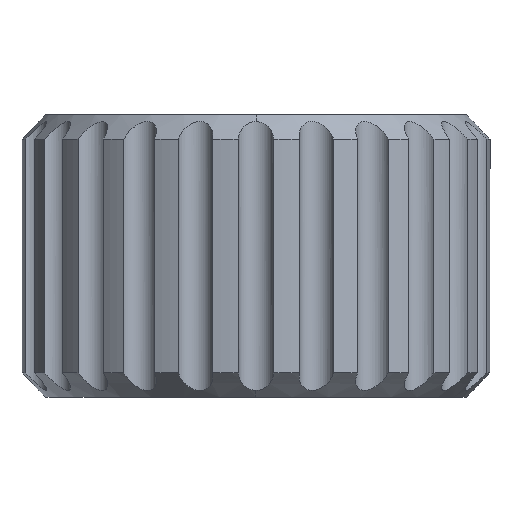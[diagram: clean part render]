
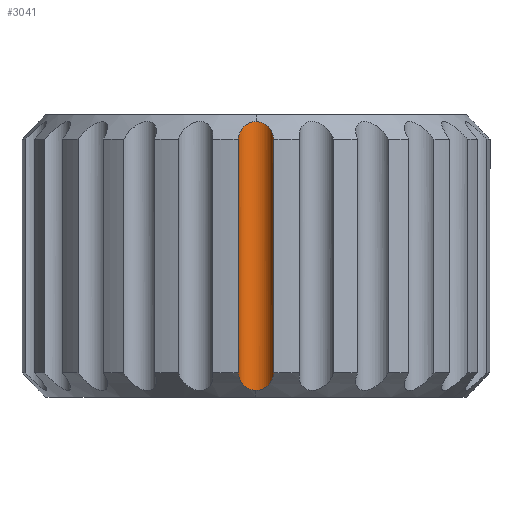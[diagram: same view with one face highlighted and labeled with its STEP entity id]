
A CAD part, front view. The second image highlights one B-rep face of the part: STEP entity #3041.
In plain terms, the highlighted cylindrical face has radius 0.635 mm (diameter 1.27 mm), a partial arc.
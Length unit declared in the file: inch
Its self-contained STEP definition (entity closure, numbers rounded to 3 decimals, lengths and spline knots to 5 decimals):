
#91 = CARTESIAN_POINT ( 'NONE',  ( -0.02498, -0.33124, -0.18272 ) ) ;
#121 = CARTESIAN_POINT ( 'NONE',  ( -0.02498, -0.33124, 0.14791 ) ) ;
#126 = CARTESIAN_POINT ( 'NONE',  ( 0., -0.30719, -0.20772 ) ) ;
#438 = CARTESIAN_POINT ( 'NONE',  ( -0.02281, -0.32026, -0.19387 ) ) ;
#469 = CARTESIAN_POINT ( 'NONE',  ( 0.00777, -0.30816, -0.20667 ) ) ;
#519 = DIRECTION ( 'NONE',  ( 0., 0., 1. ) ) ;
#771 = CARTESIAN_POINT ( 'NONE',  ( -0.0039, -0.30719, -0.20772 ) ) ;
#817 = CARTESIAN_POINT ( 'NONE',  ( -0.01414, -0.31127, -0.20334 ) ) ;
#821 = LINE ( 'NONE', #4590, #1552 ) ;
#883 = CARTESIAN_POINT ( 'NONE',  ( 0.02498, -0.33124, -0.18272 ) ) ;
#994 = CARTESIAN_POINT ( 'NONE',  ( -0.02498, -0.33124, 0.14791 ) ) ;
#1074 = ORIENTED_EDGE ( 'NONE', *, *, #4214, .T. ) ;
#1167 = CARTESIAN_POINT ( 'NONE',  ( -0.01673, -0.31336, -0.20111 ) ) ;
#1181 = CARTESIAN_POINT ( 'NONE',  ( 0.0039, -0.30719, 0.17291 ) ) ;
#1206 = VERTEX_POINT ( 'NONE', #91 ) ;
#1215 = CARTESIAN_POINT ( 'NONE',  ( 0., -0.30719, 0.17291 ) ) ;
#1312 = CARTESIAN_POINT ( 'NONE',  ( -0.02229, -0.32053, 0.15879 ) ) ;
#1376 = B_SPLINE_CURVE_WITH_KNOTS ( 'NONE', 3,
 ( #121, #2513, #2101, #1312, #4493, #3265, #2468, #2889, #3682, #3309 ),
 .UNSPECIFIED., .F., .F.,
 ( 4, 2, 2, 2, 4 ),
 ( 0., 0.0003, 0.00059, 0.00089, 0.00118 ),
 .UNSPECIFIED. ) ;
#1388 = ORIENTED_EDGE ( 'NONE', *, *, #3994, .T. ) ;
#1552 = VECTOR ( 'NONE', #3367, 39.37008 ) ;
#1601 = CARTESIAN_POINT ( 'NONE',  ( 0.0078, -0.30817, 0.17184 ) ) ;
#1610 = CARTESIAN_POINT ( 'NONE',  ( 0., -0.30719, 0.17291 ) ) ;
#1615 = CARTESIAN_POINT ( 'NONE',  ( 0.01414, -0.31127, 0.16852 ) ) ;
#1696 = AXIS2_PLACEMENT_3D ( 'NONE', #3336, #4533, #2103 ) ;
#1806 = CARTESIAN_POINT ( 'NONE',  ( 0.02498, -0.33124, -0.18272 ) ) ;
#1908 = VECTOR ( 'NONE', #519, 39.37008 ) ;
#1911 = EDGE_CURVE ( 'NONE', #2261, #3254, #1376, .T. ) ;
#1951 = CARTESIAN_POINT ( 'NONE',  ( -0.02498, -0.33124, -0.18272 ) ) ;
#1966 = CARTESIAN_POINT ( 'NONE',  ( 0., -0.30719, -0.20772 ) ) ;
#1970 = CYLINDRICAL_SURFACE ( 'NONE', #1696, 0.025 ) ;
#1986 = VERTEX_POINT ( 'NONE', #1806 ) ;
#2101 = CARTESIAN_POINT ( 'NONE',  ( -0.02432, -0.32577, 0.15342 ) ) ;
#2103 = DIRECTION ( 'NONE',  ( 1., 0., 0. ) ) ;
#2135 = CARTESIAN_POINT ( 'NONE',  ( 0.02498, -0.33124, 0.14791 ) ) ;
#2177 = ORIENTED_EDGE ( 'NONE', *, *, #4088, .F. ) ;
#2261 = VERTEX_POINT ( 'NONE', #994 ) ;
#2353 = CARTESIAN_POINT ( 'NONE',  ( -0.02477, -0.32569, -0.18828 ) ) ;
#2402 = CARTESIAN_POINT ( 'NONE',  ( 0.02432, -0.32577, -0.18824 ) ) ;
#2422 = CARTESIAN_POINT ( 'NONE',  ( 0.02281, -0.32026, 0.15905 ) ) ;
#2468 = CARTESIAN_POINT ( 'NONE',  ( -0.01417, -0.31128, 0.1685 ) ) ;
#2469 = LINE ( 'NONE', #3967, #1908 ) ;
#2513 = CARTESIAN_POINT ( 'NONE',  ( -0.02488, -0.32846, 0.15069 ) ) ;
#2651 = VERTEX_POINT ( 'NONE', #126 ) ;
#2764 = EDGE_CURVE ( 'NONE', #3254, #4951, #3009, .T. ) ;
#2796 = CARTESIAN_POINT ( 'NONE',  ( 0.01673, -0.31336, 0.16629 ) ) ;
#2889 = CARTESIAN_POINT ( 'NONE',  ( -0.00777, -0.30816, 0.17185 ) ) ;
#3009 = B_SPLINE_CURVE_WITH_KNOTS ( 'NONE', 3,
 ( #1215, #1181, #1601, #1615, #2796, #2422, #4771, #4823 ),
 .UNSPECIFIED., .F., .F.,
 ( 4, 2, 2, 4 ),
 ( 0.00118, 0.00148, 0.00177, 0.00236 ),
 .UNSPECIFIED. ) ;
#3041 = ADVANCED_FACE ( 'NONE', ( #4818 ), #1970, .F. ) ;
#3176 = EDGE_CURVE ( 'NONE', #1986, #2651, #4265, .T. ) ;
#3191 = CARTESIAN_POINT ( 'NONE',  ( 0.0039, -0.30719, -0.20772 ) ) ;
#3213 = CARTESIAN_POINT ( 'NONE',  ( 0.02488, -0.32846, -0.1855 ) ) ;
#3254 = VERTEX_POINT ( 'NONE', #1610 ) ;
#3265 = CARTESIAN_POINT ( 'NONE',  ( -0.01675, -0.31338, 0.16627 ) ) ;
#3309 = CARTESIAN_POINT ( 'NONE',  ( 0., -0.30719, 0.17291 ) ) ;
#3336 = CARTESIAN_POINT ( 'NONE',  ( 0., -0.33219, -0.23962 ) ) ;
#3367 = DIRECTION ( 'NONE',  ( 0., 0., -1. ) ) ;
#3597 = CARTESIAN_POINT ( 'NONE',  ( 0.02229, -0.32053, -0.19361 ) ) ;
#3614 = CARTESIAN_POINT ( 'NONE',  ( 0., -0.30719, -0.20772 ) ) ;
#3646 = CARTESIAN_POINT ( 'NONE',  ( 0.02079, -0.31797, -0.19626 ) ) ;
#3658 = CARTESIAN_POINT ( 'NONE',  ( 0.01675, -0.31338, -0.20109 ) ) ;
#3682 = CARTESIAN_POINT ( 'NONE',  ( -0.0039, -0.30719, 0.17291 ) ) ;
#3770 = EDGE_LOOP ( 'NONE', ( #3959, #1388, #2177, #4529, #1074, #4893 ) ) ;
#3959 = ORIENTED_EDGE ( 'NONE', *, *, #1911, .F. ) ;
#3967 = CARTESIAN_POINT ( 'NONE',  ( 0.02498, -0.33124, -0.01741 ) ) ;
#3994 = EDGE_CURVE ( 'NONE', #2261, #1206, #821, .T. ) ;
#4088 = EDGE_CURVE ( 'NONE', #2651, #1206, #4709, .T. ) ;
#4214 = EDGE_CURVE ( 'NONE', #1986, #4951, #2469, .T. ) ;
#4265 = B_SPLINE_CURVE_WITH_KNOTS ( 'NONE', 3,
 ( #883, #3213, #2402, #3597, #3646, #3658, #4849, #469, #3191, #3614 ),
 .UNSPECIFIED., .F., .F.,
 ( 4, 2, 2, 2, 4 ),
 ( 0., 0.0003, 0.00059, 0.00089, 0.00118 ),
 .UNSPECIFIED. ) ;
#4493 = CARTESIAN_POINT ( 'NONE',  ( -0.02079, -0.31797, 0.16145 ) ) ;
#4529 = ORIENTED_EDGE ( 'NONE', *, *, #3176, .F. ) ;
#4533 = DIRECTION ( 'NONE',  ( 0., 0., 1. ) ) ;
#4590 = CARTESIAN_POINT ( 'NONE',  ( -0.02498, -0.33124, -0.01741 ) ) ;
#4709 = B_SPLINE_CURVE_WITH_KNOTS ( 'NONE', 3,
 ( #1966, #771, #4774, #817, #1167, #438, #2353, #1951 ),
 .UNSPECIFIED., .F., .F.,
 ( 4, 2, 2, 4 ),
 ( 0.00118, 0.00148, 0.00177, 0.00236 ),
 .UNSPECIFIED. ) ;
#4771 = CARTESIAN_POINT ( 'NONE',  ( 0.02477, -0.32569, 0.15346 ) ) ;
#4774 = CARTESIAN_POINT ( 'NONE',  ( -0.0078, -0.30817, -0.20666 ) ) ;
#4818 = FACE_OUTER_BOUND ( 'NONE', #3770, .T. ) ;
#4823 = CARTESIAN_POINT ( 'NONE',  ( 0.02498, -0.33124, 0.14791 ) ) ;
#4849 = CARTESIAN_POINT ( 'NONE',  ( 0.01417, -0.31128, -0.20332 ) ) ;
#4893 = ORIENTED_EDGE ( 'NONE', *, *, #2764, .F. ) ;
#4951 = VERTEX_POINT ( 'NONE', #2135 ) ;
